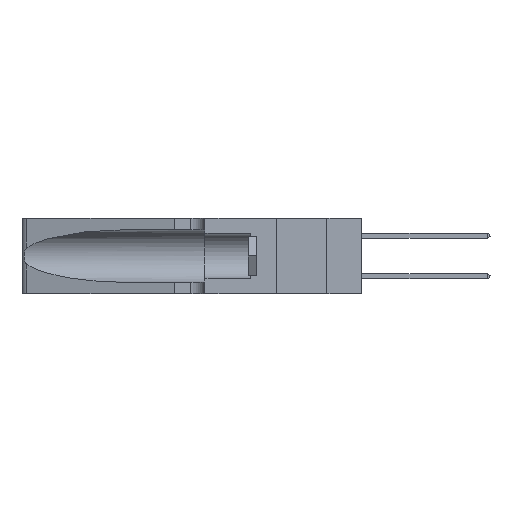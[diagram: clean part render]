
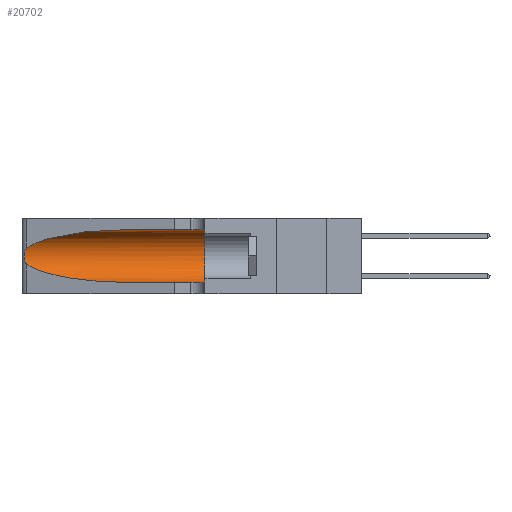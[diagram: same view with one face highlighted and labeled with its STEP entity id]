
A CAD part, left-side view. The second image highlights one B-rep face of the part: STEP entity #20702.
In plain terms, the highlighted cylindrical face has radius 3.308 mm (diameter 6.617 mm), a partial arc.
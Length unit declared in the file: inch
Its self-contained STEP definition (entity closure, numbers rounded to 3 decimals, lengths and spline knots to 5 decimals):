
#114 = EDGE_CURVE ( 'NONE', #20338, #31948, #25040, .T. ) ;
#829 = CARTESIAN_POINT ( 'NONE',  ( 0.26075, 1.23896, 0.19203 ) ) ;
#1183 = AXIS2_PLACEMENT_3D ( 'NONE', #14215, #35711, #17324 ) ;
#1495 = VERTEX_POINT ( 'NONE', #15766 ) ;
#1764 = CARTESIAN_POINT ( 'NONE',  ( 0.25487, 1.22718, 0.22369 ) ) ;
#2446 = DIRECTION ( 'NONE',  ( 0., -1., 0. ) ) ;
#3002 = ORIENTED_EDGE ( 'NONE', *, *, #38673, .F. ) ;
#3145 = CARTESIAN_POINT ( 'NONE',  ( 0.1305, 0.72297, 0.31525 ) ) ;
#3540 = CARTESIAN_POINT ( 'NONE',  ( 0.1305, 0.35, 0.05475 ) ) ;
#3722 = CARTESIAN_POINT ( 'NONE',  ( 0.2373, 1.15595, 0.08982 ) ) ;
#3913 = CARTESIAN_POINT ( 'NONE',  ( 0.26017, 1.23833, 0.17102 ) ) ;
#5480 = CARTESIAN_POINT ( 'NONE',  ( 0.1305, 1.61858, 0.05475 ) ) ;
#6791 = EDGE_CURVE ( 'NONE', #1495, #20256, #8199, .T. ) ;
#6866 = CARTESIAN_POINT ( 'NONE',  ( 0.25555, 1.22994, 0.2215 ) ) ;
#6899 = CARTESIAN_POINT ( 'NONE',  ( 0.1305, 0.72297, 0.31525 ) ) ;
#6997 = CARTESIAN_POINT ( 'NONE',  ( 0.25789, 1.23486, 0.15765 ) ) ;
#8199 = CIRCLE ( 'NONE', #1183, 0.13025 ) ;
#8503 = CYLINDRICAL_SURFACE ( 'NONE', #14565, 0.13025 ) ;
#8889 = ORIENTED_EDGE ( 'NONE', *, *, #24241, .T. ) ;
#9493 = B_SPLINE_CURVE_WITH_KNOTS ( 'NONE', 3,
 ( #34405, #6866, #34532, #16174, #37675, #19282, #829, #22404, #3913, #25446, #6997, #28531, #10095, #31620 ),
 .UNSPECIFIED., .F., .F.,
 ( 4, 2, 2, 2, 2, 2, 4 ),
 ( 0., 0.00027, 0.00053, 0.00107, 0.0016, 0.00187, 0.00214 ),
 .UNSPECIFIED. ) ;
#9518 = CARTESIAN_POINT ( 'NONE',  ( 0.25487, 1.22718, 0.14631 ) ) ;
#10095 = CARTESIAN_POINT ( 'NONE',  ( 0.25555, 1.22993, 0.14849 ) ) ;
#11095 = VECTOR ( 'NONE', #30103, 39.37008 ) ;
#12071 = LINE ( 'NONE', #5480, #11095 ) ;
#12177 = CARTESIAN_POINT ( 'NONE',  ( 0.2373, 1.15595, 0.28018 ) ) ;
#13012 = CARTESIAN_POINT ( 'NONE',  ( 0.1305, 0.72297, 0.05475 ) ) ;
#13939 = VERTEX_POINT ( 'NONE', #9518 ) ;
#14215 = CARTESIAN_POINT ( 'NONE',  ( 0.1305, 0.35, 0.185 ) ) ;
#14565 = AXIS2_PLACEMENT_3D ( 'NONE', #20948, #2446, #39293 ) ;
#15766 = CARTESIAN_POINT ( 'NONE',  ( 0.1305, 0.35, 0.31525 ) ) ;
#16174 = CARTESIAN_POINT ( 'NONE',  ( 0.25787, 1.23484, 0.2124 ) ) ;
#16321 = EDGE_CURVE ( 'NONE', #13939, #26170, #23848, .T. ) ;
#16547 = VECTOR ( 'NONE', #37339, 39.37008 ) ;
#17016 = CARTESIAN_POINT ( 'NONE',  ( 0.18966, 0.96281, 0.31525 ) ) ;
#17324 = DIRECTION ( 'NONE',  ( 0., 0., 1. ) ) ;
#17681 = ORIENTED_EDGE ( 'NONE', *, *, #16321, .T. ) ;
#19282 = CARTESIAN_POINT ( 'NONE',  ( 0.26018, 1.23835, 0.19895 ) ) ;
#20256 = VERTEX_POINT ( 'NONE', #3540 ) ;
#20338 = VERTEX_POINT ( 'NONE', #6899 ) ;
#20702 = ADVANCED_FACE ( 'NONE', ( #33038 ), #8503, .F. ) ;
#20897 = EDGE_CURVE ( 'NONE', #31948, #13939, #9493, .T. ) ;
#20948 = CARTESIAN_POINT ( 'NONE',  ( 0.1305, 1.61858, 0.185 ) ) ;
#21777 = CARTESIAN_POINT ( 'NONE',  ( 0.25487, 1.22718, 0.22369 ) ) ;
#22404 = CARTESIAN_POINT ( 'NONE',  ( 0.26075, 1.23896, 0.178 ) ) ;
#22584 = ORIENTED_EDGE ( 'NONE', *, *, #20897, .T. ) ;
#22828 = LINE ( 'NONE', #34206, #16547 ) ;
#23848 =( BOUNDED_CURVE ( )  B_SPLINE_CURVE ( 3, ( #28333, #3722, #31439, #13012 ),
 .UNSPECIFIED., .F., .F. ) 
 B_SPLINE_CURVE_WITH_KNOTS ( ( 4, 4 ),
 ( 3.44316, 4.71239 ),
 .UNSPECIFIED. ) 
 CURVE ( )  GEOMETRIC_REPRESENTATION_ITEM ( )  RATIONAL_B_SPLINE_CURVE ( ( 1., 0.87, 0.87, 1. ) ) 
 REPRESENTATION_ITEM ( '' )  );
#23990 = ORIENTED_EDGE ( 'NONE', *, *, #114, .T. ) ;
#24241 = EDGE_CURVE ( 'NONE', #26170, #20256, #12071, .T. ) ;
#25040 =( BOUNDED_CURVE ( )  B_SPLINE_CURVE ( 3, ( #3145, #17016, #12177, #21777 ),
 .UNSPECIFIED., .F., .F. ) 
 B_SPLINE_CURVE_WITH_KNOTS ( ( 4, 4 ),
 ( 1.5708, 2.84003 ),
 .UNSPECIFIED. ) 
 CURVE ( )  GEOMETRIC_REPRESENTATION_ITEM ( )  RATIONAL_B_SPLINE_CURVE ( ( 1., 0.87, 0.87, 1. ) ) 
 REPRESENTATION_ITEM ( '' )  );
#25446 = CARTESIAN_POINT ( 'NONE',  ( 0.25856, 1.23593, 0.16098 ) ) ;
#26170 = VERTEX_POINT ( 'NONE', #35270 ) ;
#28333 = CARTESIAN_POINT ( 'NONE',  ( 0.25487, 1.22718, 0.14631 ) ) ;
#28531 = CARTESIAN_POINT ( 'NONE',  ( 0.25639, 1.23186, 0.15144 ) ) ;
#30080 = ORIENTED_EDGE ( 'NONE', *, *, #6791, .F. ) ;
#30103 = DIRECTION ( 'NONE',  ( 0., -1., 0. ) ) ;
#31439 = CARTESIAN_POINT ( 'NONE',  ( 0.18966, 0.96281, 0.05475 ) ) ;
#31620 = CARTESIAN_POINT ( 'NONE',  ( 0.25487, 1.22718, 0.14631 ) ) ;
#31948 = VERTEX_POINT ( 'NONE', #1764 ) ;
#33038 = FACE_OUTER_BOUND ( 'NONE', #33711, .T. ) ;
#33711 = EDGE_LOOP ( 'NONE', ( #23990, #22584, #17681, #8889, #30080, #3002 ) ) ;
#34206 = CARTESIAN_POINT ( 'NONE',  ( 0.1305, 1.61858, 0.31525 ) ) ;
#34405 = CARTESIAN_POINT ( 'NONE',  ( 0.25487, 1.22718, 0.22369 ) ) ;
#34532 = CARTESIAN_POINT ( 'NONE',  ( 0.25639, 1.23184, 0.21858 ) ) ;
#35270 = CARTESIAN_POINT ( 'NONE',  ( 0.1305, 0.72297, 0.05475 ) ) ;
#35711 = DIRECTION ( 'NONE',  ( 0., 1., 0. ) ) ;
#37339 = DIRECTION ( 'NONE',  ( 0., -1., 0. ) ) ;
#37675 = CARTESIAN_POINT ( 'NONE',  ( 0.25854, 1.2359, 0.20912 ) ) ;
#38673 = EDGE_CURVE ( 'NONE', #20338, #1495, #22828, .T. ) ;
#39293 = DIRECTION ( 'NONE',  ( 0., 0., -1. ) ) ;
